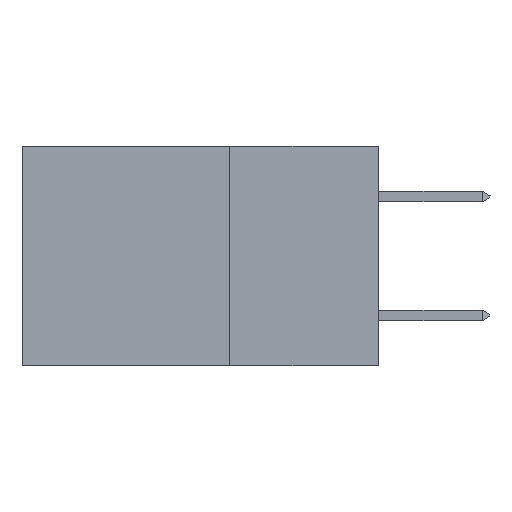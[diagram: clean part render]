
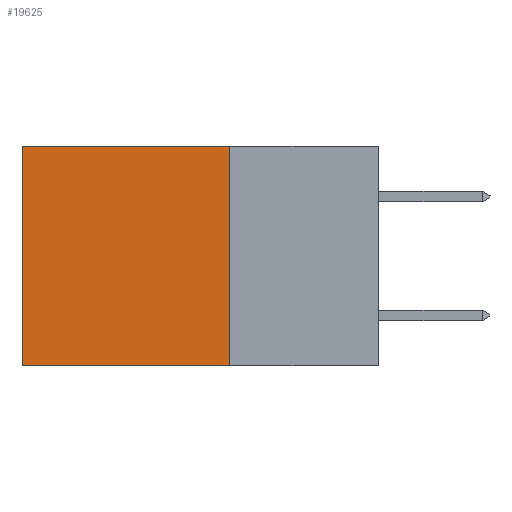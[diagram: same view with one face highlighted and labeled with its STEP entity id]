
A CAD part, left-side view. The second image highlights one B-rep face of the part: STEP entity #19625.
In plain terms, the highlighted planar face has unit normal (-1, 0, 0).
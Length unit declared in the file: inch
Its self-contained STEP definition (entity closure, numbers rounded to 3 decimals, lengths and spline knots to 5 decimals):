
#2229 = EDGE_LOOP ( 'NONE', ( #16573, #6849, #18363, #13340 ) ) ;
#3422 = VECTOR ( 'NONE', #14575, 39.37008 ) ;
#3818 = DIRECTION ( 'NONE',  ( 1., 0., 0. ) ) ;
#6090 = EDGE_CURVE ( 'NONE', #14071, #21773, #7856, .T. ) ;
#6589 = DIRECTION ( 'NONE',  ( 0., 1., 0. ) ) ;
#6849 = ORIENTED_EDGE ( 'NONE', *, *, #14266, .F. ) ;
#7364 = PLANE ( 'NONE',  #10794 ) ;
#7856 = LINE ( 'NONE', #13373, #15098 ) ;
#8235 = CARTESIAN_POINT ( 'NONE',  ( 0.2615, 0.25, -0.37 ) ) ;
#8654 = EDGE_CURVE ( 'NONE', #21773, #8909, #18249, .T. ) ;
#8846 = CARTESIAN_POINT ( 'NONE',  ( 0.2615, 0.6, 0. ) ) ;
#8909 = VERTEX_POINT ( 'NONE', #19255 ) ;
#9423 = VERTEX_POINT ( 'NONE', #10485 ) ;
#10485 = CARTESIAN_POINT ( 'NONE',  ( 0.2615, 0.25, -0.37 ) ) ;
#10794 = AXIS2_PLACEMENT_3D ( 'NONE', #19548, #3818, #14383 ) ;
#12071 = VECTOR ( 'NONE', #6589, 39.37008 ) ;
#13340 = ORIENTED_EDGE ( 'NONE', *, *, #6090, .T. ) ;
#13373 = CARTESIAN_POINT ( 'NONE',  ( 0.2615, 0.25, 0. ) ) ;
#14071 = VERTEX_POINT ( 'NONE', #22215 ) ;
#14266 = EDGE_CURVE ( 'NONE', #9423, #8909, #19120, .T. ) ;
#14383 = DIRECTION ( 'NONE',  ( 0., 0., -1. ) ) ;
#14575 = DIRECTION ( 'NONE',  ( 0., 0., -1. ) ) ;
#14820 = LINE ( 'NONE', #8235, #15030 ) ;
#15030 = VECTOR ( 'NONE', #18053, 39.37008 ) ;
#15044 = EDGE_CURVE ( 'NONE', #14071, #9423, #14820, .T. ) ;
#15098 = VECTOR ( 'NONE', #16605, 39.37008 ) ;
#15798 = CARTESIAN_POINT ( 'NONE',  ( 0.2615, 0.25, -0.37 ) ) ;
#16530 = CARTESIAN_POINT ( 'NONE',  ( 0.2615, 0.6, -0.37 ) ) ;
#16573 = ORIENTED_EDGE ( 'NONE', *, *, #8654, .T. ) ;
#16605 = DIRECTION ( 'NONE',  ( 0., 1., 0. ) ) ;
#18053 = DIRECTION ( 'NONE',  ( 0., 0., -1. ) ) ;
#18249 = LINE ( 'NONE', #16530, #3422 ) ;
#18363 = ORIENTED_EDGE ( 'NONE', *, *, #15044, .F. ) ;
#19120 = LINE ( 'NONE', #15798, #12071 ) ;
#19255 = CARTESIAN_POINT ( 'NONE',  ( 0.2615, 0.6, -0.37 ) ) ;
#19548 = CARTESIAN_POINT ( 'NONE',  ( 0.2615, 0.25, -0.37 ) ) ;
#19625 = ADVANCED_FACE ( 'NONE', ( #19651 ), #7364, .F. ) ;
#19651 = FACE_OUTER_BOUND ( 'NONE', #2229, .T. ) ;
#21773 = VERTEX_POINT ( 'NONE', #8846 ) ;
#22215 = CARTESIAN_POINT ( 'NONE',  ( 0.2615, 0.25, 0. ) ) ;
